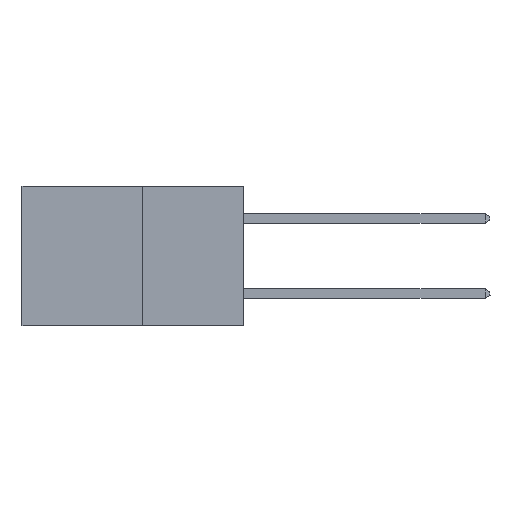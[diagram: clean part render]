
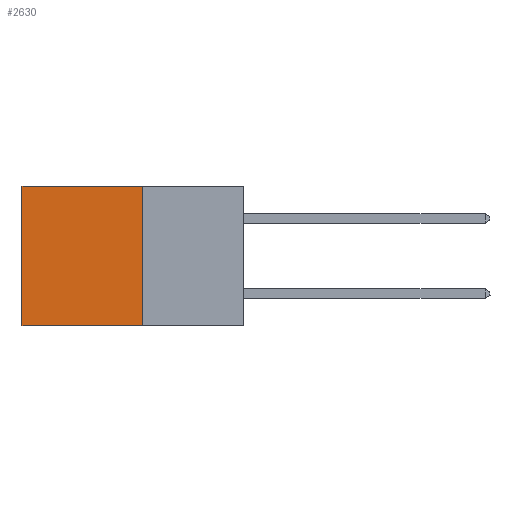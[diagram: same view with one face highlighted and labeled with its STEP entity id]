
A CAD part, left-side view. The second image highlights one B-rep face of the part: STEP entity #2630.
In plain terms, the highlighted planar face has unit normal (-1, 0, 0).
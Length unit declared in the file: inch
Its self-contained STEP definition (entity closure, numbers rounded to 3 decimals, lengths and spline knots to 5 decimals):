
#324 = AXIS2_PLACEMENT_3D ( 'NONE', #9109, #8371, #8405 ) ;
#794 = DIRECTION ( 'NONE',  ( 0., 0., -1. ) ) ;
#1419 = CARTESIAN_POINT ( 'NONE',  ( 0.277, 0.27, -0.37 ) ) ;
#2136 = LINE ( 'NONE', #1419, #10899 ) ;
#2431 = LINE ( 'NONE', #9396, #8445 ) ;
#2630 = ADVANCED_FACE ( 'NONE', ( #6682 ), #10259, .F. ) ;
#2944 = VECTOR ( 'NONE', #5914, 39.37008 ) ;
#3107 = VERTEX_POINT ( 'NONE', #6916 ) ;
#3481 = CARTESIAN_POINT ( 'NONE',  ( 0.277, 0.27, 0. ) ) ;
#3674 = VERTEX_POINT ( 'NONE', #10106 ) ;
#3774 = DIRECTION ( 'NONE',  ( 0., 1., 0. ) ) ;
#3937 = EDGE_LOOP ( 'NONE', ( #9006, #7840, #4349, #7153 ) ) ;
#4349 = ORIENTED_EDGE ( 'NONE', *, *, #7193, .F. ) ;
#4549 = CARTESIAN_POINT ( 'NONE',  ( 0.277, 0.27, 0. ) ) ;
#5410 = VECTOR ( 'NONE', #3774, 39.37008 ) ;
#5527 = EDGE_CURVE ( 'NONE', #8883, #10360, #5673, .T. ) ;
#5673 = LINE ( 'NONE', #4549, #5410 ) ;
#5869 = EDGE_CURVE ( 'NONE', #10360, #3107, #2431, .T. ) ;
#5914 = DIRECTION ( 'NONE',  ( 0., 1., 0. ) ) ;
#6037 = CARTESIAN_POINT ( 'NONE',  ( 0.277, 0.27, -0.37 ) ) ;
#6177 = EDGE_CURVE ( 'NONE', #3674, #3107, #7526, .T. ) ;
#6235 = CARTESIAN_POINT ( 'NONE',  ( 0.277, 0.59, 0. ) ) ;
#6682 = FACE_OUTER_BOUND ( 'NONE', #3937, .T. ) ;
#6916 = CARTESIAN_POINT ( 'NONE',  ( 0.277, 0.59, -0.37 ) ) ;
#7153 = ORIENTED_EDGE ( 'NONE', *, *, #5527, .T. ) ;
#7193 = EDGE_CURVE ( 'NONE', #8883, #3674, #2136, .T. ) ;
#7526 = LINE ( 'NONE', #6037, #2944 ) ;
#7840 = ORIENTED_EDGE ( 'NONE', *, *, #6177, .F. ) ;
#8371 = DIRECTION ( 'NONE',  ( 1., 0., 0. ) ) ;
#8405 = DIRECTION ( 'NONE',  ( 0., 0., -1. ) ) ;
#8445 = VECTOR ( 'NONE', #9001, 39.37008 ) ;
#8883 = VERTEX_POINT ( 'NONE', #3481 ) ;
#9001 = DIRECTION ( 'NONE',  ( 0., 0., -1. ) ) ;
#9006 = ORIENTED_EDGE ( 'NONE', *, *, #5869, .T. ) ;
#9109 = CARTESIAN_POINT ( 'NONE',  ( 0.277, 0.27, -0.37 ) ) ;
#9396 = CARTESIAN_POINT ( 'NONE',  ( 0.277, 0.59, -0.37 ) ) ;
#10106 = CARTESIAN_POINT ( 'NONE',  ( 0.277, 0.27, -0.37 ) ) ;
#10259 = PLANE ( 'NONE',  #324 ) ;
#10360 = VERTEX_POINT ( 'NONE', #6235 ) ;
#10899 = VECTOR ( 'NONE', #794, 39.37008 ) ;
